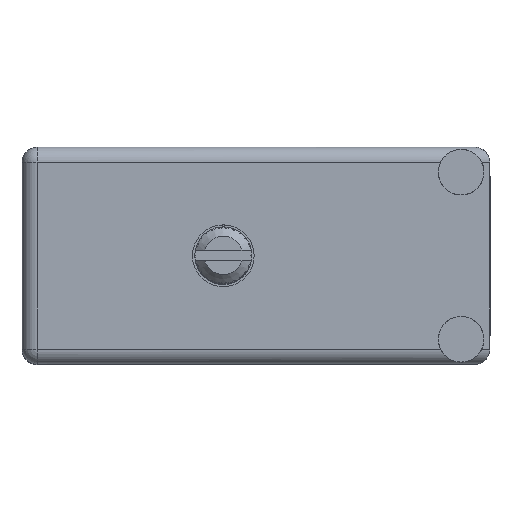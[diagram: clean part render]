
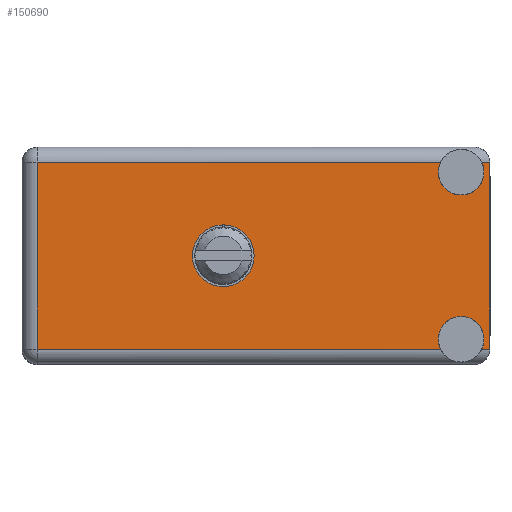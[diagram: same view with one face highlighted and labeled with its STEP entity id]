
A CAD part, top view. The second image highlights one B-rep face of the part: STEP entity #150690.
In plain terms, the highlighted face is planar.
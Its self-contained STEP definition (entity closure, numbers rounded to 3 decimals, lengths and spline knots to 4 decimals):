
#1027 = ORIENTED_EDGE ( 'NONE', *, *, #39023, .F. ) ;
#3101 = CIRCLE ( 'NONE', #60136, 0.075 ) ;
#4893 = VERTEX_POINT ( 'NONE', #185910 ) ;
#6719 = CARTESIAN_POINT ( 'NONE',  ( 0., 0.906, -0.715 ) ) ;
#7943 = VECTOR ( 'NONE', #142396, 39.3701 ) ;
#9282 = ORIENTED_EDGE ( 'NONE', *, *, #95872, .T. ) ;
#11033 = EDGE_CURVE ( 'NONE', #33156, #78578, #11660, .T. ) ;
#11660 = LINE ( 'NONE', #125457, #159794 ) ;
#15281 = DIRECTION ( 'NONE',  ( 0., 0., 1. ) ) ;
#15544 = DIRECTION ( 'NONE',  ( 0., 0., 1. ) ) ;
#18261 = VECTOR ( 'NONE', #113211, 39.3701 ) ;
#19619 = ORIENTED_EDGE ( 'NONE', *, *, #173951, .F. ) ;
#20680 = ORIENTED_EDGE ( 'NONE', *, *, #74631, .T. ) ;
#21602 = DIRECTION ( 'NONE',  ( 1., 0., 0. ) ) ;
#22085 = DIRECTION ( 'NONE',  ( -1., 0., 0. ) ) ;
#23006 = DIRECTION ( 'NONE',  ( 0., 1., 0. ) ) ;
#24928 = LINE ( 'NONE', #125510, #7943 ) ;
#26660 = VECTOR ( 'NONE', #22085, 39.3701 ) ;
#27185 = CARTESIAN_POINT ( 'NONE',  ( 1.539, 0.906, -0.665 ) ) ;
#33156 = VERTEX_POINT ( 'NONE', #175049 ) ;
#33356 = LINE ( 'NONE', #115229, #148882 ) ;
#35230 = EDGE_CURVE ( 'NONE', #112294, #33156, #144197, .T. ) ;
#36515 = CIRCLE ( 'NONE', #126591, 0.075 ) ;
#37971 = EDGE_LOOP ( 'NONE', ( #140828, #180507, #19619, #41134, #121809, #20680, #91428, #1027, #9282, #54446 ) ) ;
#38009 = CARTESIAN_POINT ( 'NONE',  ( 0.6625, 0.906, -0.459 ) ) ;
#39023 = EDGE_CURVE ( 'NONE', #176468, #137071, #3101, .T. ) ;
#40499 = CARTESIAN_POINT ( 'NONE',  ( 1.445, 0.906, -0.0825 ) ) ;
#41134 = ORIENTED_EDGE ( 'NONE', *, *, #181393, .T. ) ;
#44966 = CARTESIAN_POINT ( 'NONE',  ( 1.3774, 0.906, -0.05 ) ) ;
#45555 = AXIS2_PLACEMENT_3D ( 'NONE', #6719, #107307, #164678 ) ;
#46441 = ORIENTED_EDGE ( 'NONE', *, *, #75275, .F. ) ;
#47046 = LINE ( 'NONE', #118494, #51962 ) ;
#49054 = FACE_BOUND ( 'NONE', #54595, .T. ) ;
#51962 = VECTOR ( 'NONE', #21602, 39.3701 ) ;
#54412 = CARTESIAN_POINT ( 'NONE',  ( 1.445, 0.906, -0.1575 ) ) ;
#54446 = ORIENTED_EDGE ( 'NONE', *, *, #35230, .T. ) ;
#54595 = EDGE_LOOP ( 'NONE', ( #177283, #46441 ) ) ;
#60136 = AXIS2_PLACEMENT_3D ( 'NONE', #86753, #87665, #76316 ) ;
#62973 = CARTESIAN_POINT ( 'NONE',  ( 1.5126, 0.906, -0.665 ) ) ;
#66544 = CARTESIAN_POINT ( 'NONE',  ( 1.445, 0.906, -0.6325 ) ) ;
#68078 = LINE ( 'NONE', #125463, #26660 ) ;
#74631 = EDGE_CURVE ( 'NONE', #109070, #141528, #24928, .T. ) ;
#75275 = EDGE_CURVE ( 'NONE', #166883, #145480, #155085, .T. ) ;
#76316 = DIRECTION ( 'NONE',  ( 0., 0., 1. ) ) ;
#78578 = VERTEX_POINT ( 'NONE', #44966 ) ;
#81054 = EDGE_CURVE ( 'NONE', #90818, #78578, #122310, .T. ) ;
#84423 = CARTESIAN_POINT ( 'NONE',  ( 1.445, 0.906, -0.5575 ) ) ;
#86753 = CARTESIAN_POINT ( 'NONE',  ( 1.445, 0.906, -0.6325 ) ) ;
#87665 = DIRECTION ( 'NONE',  ( 0., 1., 0. ) ) ;
#90818 = VERTEX_POINT ( 'NONE', #54412 ) ;
#91428 = ORIENTED_EDGE ( 'NONE', *, *, #134962, .F. ) ;
#95443 = CARTESIAN_POINT ( 'NONE',  ( 1.5126, 0.906, -0.05 ) ) ;
#95872 = EDGE_CURVE ( 'NONE', #176468, #112294, #68078, .T. ) ;
#102712 = CARTESIAN_POINT ( 'NONE',  ( 1.445, 0.906, -0.0825 ) ) ;
#105639 = EDGE_CURVE ( 'NONE', #109070, #4893, #33356, .T. ) ;
#107307 = DIRECTION ( 'NONE',  ( 0., 1., 0. ) ) ;
#109070 = VERTEX_POINT ( 'NONE', #27185 ) ;
#111358 = DIRECTION ( 'NONE',  ( 1., 0., 0. ) ) ;
#112294 = VERTEX_POINT ( 'NONE', #176948 ) ;
#113211 = DIRECTION ( 'NONE',  ( 0., 0., 1. ) ) ;
#115229 = CARTESIAN_POINT ( 'NONE',  ( 1.539, 0.906, 0. ) ) ;
#118494 = CARTESIAN_POINT ( 'NONE',  ( 1.539, 0.906, -0.05 ) ) ;
#118657 = DIRECTION ( 'NONE',  ( 0., 1., 0. ) ) ;
#121556 = CARTESIAN_POINT ( 'NONE',  ( 0.6625, 0.906, -0.3575 ) ) ;
#121731 = CARTESIAN_POINT ( 'NONE',  ( 0.6625, 0.906, -0.3575 ) ) ;
#121809 = ORIENTED_EDGE ( 'NONE', *, *, #105639, .F. ) ;
#122310 = CIRCLE ( 'NONE', #185415, 0.075 ) ;
#123274 = DIRECTION ( 'NONE',  ( 0., 0., 1. ) ) ;
#125457 = CARTESIAN_POINT ( 'NONE',  ( 1.539, 0.906, -0.05 ) ) ;
#125463 = CARTESIAN_POINT ( 'NONE',  ( 0., 0.906, -0.665 ) ) ;
#125510 = CARTESIAN_POINT ( 'NONE',  ( 0., 0.906, -0.665 ) ) ;
#126591 = AXIS2_PLACEMENT_3D ( 'NONE', #102712, #118657, #15281 ) ;
#129255 = CARTESIAN_POINT ( 'NONE',  ( 1.3774, 0.906, -0.665 ) ) ;
#132895 = DIRECTION ( 'NONE',  ( 0., 0., 1. ) ) ;
#134962 = EDGE_CURVE ( 'NONE', #137071, #141528, #162203, .T. ) ;
#135540 = FACE_OUTER_BOUND ( 'NONE', #37971, .T. ) ;
#137071 = VERTEX_POINT ( 'NONE', #84423 ) ;
#137070 = AXIS2_PLACEMENT_3D ( 'NONE', #121556, #147909, #132895 ) ;
#138297 = DIRECTION ( 'NONE',  ( 0., 1., 0. ) ) ;
#138413 = CARTESIAN_POINT ( 'NONE',  ( 0.6625, 0.906, -0.256 ) ) ;
#140828 = ORIENTED_EDGE ( 'NONE', *, *, #11033, .T. ) ;
#141528 = VERTEX_POINT ( 'NONE', #62973 ) ;
#142346 = CARTESIAN_POINT ( 'NONE',  ( 0.05, 0.906, -0.715 ) ) ;
#142396 = DIRECTION ( 'NONE',  ( -1., 0., 0. ) ) ;
#144197 = LINE ( 'NONE', #142346, #18261 ) ;
#145480 = VERTEX_POINT ( 'NONE', #138413 ) ;
#147909 = DIRECTION ( 'NONE',  ( 0., 1., 0. ) ) ;
#148882 = VECTOR ( 'NONE', #15544, 39.3701 ) ;
#150690 = ADVANCED_FACE ( 'NONE', ( #49054, #135540 ), #163760, .T. ) ;
#152940 = EDGE_CURVE ( 'NONE', #145480, #166883, #183830, .T. ) ;
#155085 = CIRCLE ( 'NONE', #137070, 0.1015 ) ;
#159794 = VECTOR ( 'NONE', #111358, 39.3701 ) ;
#162203 = CIRCLE ( 'NONE', #174181, 0.075 ) ;
#163760 = PLANE ( 'NONE',  #45555 ) ;
#164678 = DIRECTION ( 'NONE',  ( 0., 0., 1. ) ) ;
#166883 = VERTEX_POINT ( 'NONE', #38009 ) ;
#171890 = AXIS2_PLACEMENT_3D ( 'NONE', #121731, #23006, #178213 ) ;
#173951 = EDGE_CURVE ( 'NONE', #182396, #90818, #36515, .T. ) ;
#174181 = AXIS2_PLACEMENT_3D ( 'NONE', #66544, #182227, #183166 ) ;
#175049 = CARTESIAN_POINT ( 'NONE',  ( 0.05, 0.906, -0.05 ) ) ;
#176468 = VERTEX_POINT ( 'NONE', #129255 ) ;
#176948 = CARTESIAN_POINT ( 'NONE',  ( 0.05, 0.906, -0.665 ) ) ;
#177283 = ORIENTED_EDGE ( 'NONE', *, *, #152940, .F. ) ;
#178213 = DIRECTION ( 'NONE',  ( 0., 0., 1. ) ) ;
#180507 = ORIENTED_EDGE ( 'NONE', *, *, #81054, .F. ) ;
#181393 = EDGE_CURVE ( 'NONE', #182396, #4893, #47046, .T. ) ;
#182227 = DIRECTION ( 'NONE',  ( 0., 1., 0. ) ) ;
#182396 = VERTEX_POINT ( 'NONE', #95443 ) ;
#183166 = DIRECTION ( 'NONE',  ( 0., 0., 1. ) ) ;
#183830 = CIRCLE ( 'NONE', #171890, 0.1015 ) ;
#185415 = AXIS2_PLACEMENT_3D ( 'NONE', #40499, #138297, #123274 ) ;
#185910 = CARTESIAN_POINT ( 'NONE',  ( 1.539, 0.906, -0.05 ) ) ;
